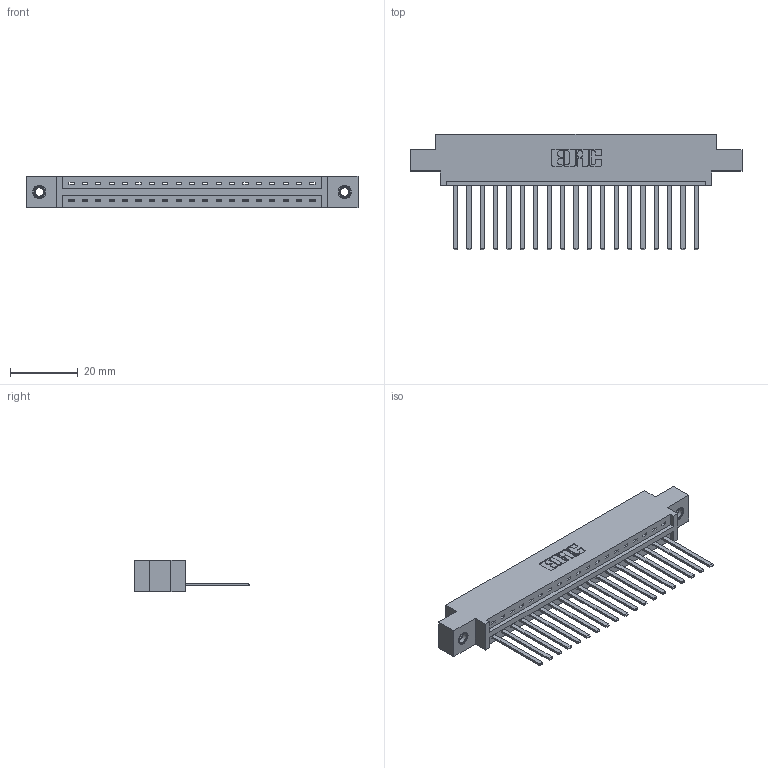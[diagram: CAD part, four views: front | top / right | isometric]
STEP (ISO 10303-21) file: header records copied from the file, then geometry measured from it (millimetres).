
FILE_DESCRIPTION (( 'STEP AP203' ), '1' );
FILE_NAME ('387-019-544-607.STEP', '2019-10-02T21:50:21', ( '' ), ( '' ), 'SwSTEP 2.0', 'SolidWorks 2016', '' );
FILE_SCHEMA (( 'CONFIG_CONTROL_DESIGN' ));
Length unit declared in the file: inch
Products named in the file (4): 345-292-001_345-293-144; 387-019-544-607; 345-250-001_345-250-005-103; 337 Part_0.170 Offset - 0.156 Dia-TI
Assembly tree (22 placements, depth 2):
  387-019-544-607
    337 Part_0.170 Offset - 0.156 Dia-TI
    345-292-001_345-293-144  x19
    345-250-001_345-250-005-103  x2
Bounding box: 98.3 x 34.3 x 9.4 mm (x, y, z)
Volume: 10017.6 mm3; surface area: 11085.4 mm2
Topology: 22 solids, 22 shells, 1242 faces, 3689 edges, 2426 vertices
Faces by surface type: plane 904, cylinder 322, cone 12, torus 4
Entity records: 18232 total; most frequent: CARTESIAN_POINT 3154, ORIENTED_EDGE 3102, DIRECTION 2731, EDGE_CURVE 1551, VECTOR 1407, LINE 1407, VERTEX_POINT 1028, AXIS2_PLACEMENT_3D 662
